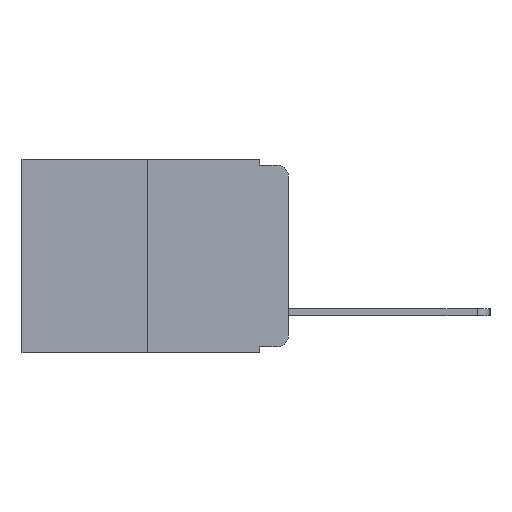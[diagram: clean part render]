
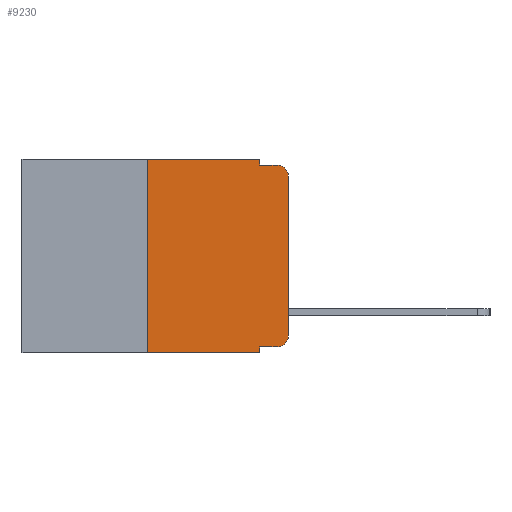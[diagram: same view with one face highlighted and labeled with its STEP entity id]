
A CAD part, left-side view. The second image highlights one B-rep face of the part: STEP entity #9230.
In plain terms, the highlighted planar face has unit normal (-1, 0, 0).
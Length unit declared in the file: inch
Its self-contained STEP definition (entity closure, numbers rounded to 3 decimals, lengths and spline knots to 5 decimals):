
#603 = VECTOR ( 'NONE', #9681, 39.37008 ) ;
#700 = AXIS2_PLACEMENT_3D ( 'NONE', #1759, #1698, #7909 ) ;
#852 = EDGE_CURVE ( 'NONE', #17246, #5633, #21928, .T. ) ;
#853 = CARTESIAN_POINT ( 'NONE',  ( 0., 0.051, -0.333 ) ) ;
#1263 = LINE ( 'NONE', #16762, #5682 ) ;
#1351 = VERTEX_POINT ( 'NONE', #10596 ) ;
#1698 = DIRECTION ( 'NONE',  ( -1., 0., 0. ) ) ;
#1759 = CARTESIAN_POINT ( 'NONE',  ( 0., 0.02, -0.313 ) ) ;
#2240 = EDGE_CURVE ( 'NONE', #18007, #17246, #8905, .T. ) ;
#2505 = LINE ( 'NONE', #14826, #11472 ) ;
#2826 = VERTEX_POINT ( 'NONE', #3504 ) ;
#2918 = LINE ( 'NONE', #5590, #16963 ) ;
#3504 = CARTESIAN_POINT ( 'NONE',  ( 0., 0.051, -0.343 ) ) ;
#3516 = EDGE_CURVE ( 'NONE', #18007, #2826, #2918, .T. ) ;
#4063 = ORIENTED_EDGE ( 'NONE', *, *, #4723, .F. ) ;
#4288 = DIRECTION ( 'NONE',  ( 0., -1., 0. ) ) ;
#4389 = CARTESIAN_POINT ( 'NONE',  ( 0., 0.25, -0.343 ) ) ;
#4510 = DIRECTION ( 'NONE',  ( 0., 0., 1. ) ) ;
#4723 = EDGE_CURVE ( 'NONE', #5943, #1351, #1263, .T. ) ;
#4977 = VERTEX_POINT ( 'NONE', #5205 ) ;
#5091 = ORIENTED_EDGE ( 'NONE', *, *, #3516, .F. ) ;
#5205 = CARTESIAN_POINT ( 'NONE',  ( 0., 0.051, -0.01 ) ) ;
#5473 = VERTEX_POINT ( 'NONE', #18615 ) ;
#5590 = CARTESIAN_POINT ( 'NONE',  ( 0., 0.051, 0. ) ) ;
#5633 = VERTEX_POINT ( 'NONE', #17326 ) ;
#5682 = VECTOR ( 'NONE', #4510, 39.37008 ) ;
#5930 = EDGE_CURVE ( 'NONE', #6834, #4977, #14478, .T. ) ;
#5943 = VERTEX_POINT ( 'NONE', #4389 ) ;
#6155 = CARTESIAN_POINT ( 'NONE',  ( 0., 0.473, 0. ) ) ;
#6527 = EDGE_CURVE ( 'NONE', #1351, #6834, #2505, .T. ) ;
#6761 = CARTESIAN_POINT ( 'NONE',  ( 0., 0.051, 0. ) ) ;
#6834 = VERTEX_POINT ( 'NONE', #6761 ) ;
#7132 = EDGE_CURVE ( 'NONE', #4977, #5473, #13359, .T. ) ;
#7755 = LINE ( 'NONE', #14783, #11308 ) ;
#7909 = DIRECTION ( 'NONE',  ( 0., 0., -1. ) ) ;
#7927 = CARTESIAN_POINT ( 'NONE',  ( 0., 0.051, 0. ) ) ;
#8905 = LINE ( 'NONE', #10770, #22115 ) ;
#9230 = ADVANCED_FACE ( 'NONE', ( #16764 ), #9718, .F. ) ;
#9500 = EDGE_CURVE ( 'NONE', #19135, #5473, #15961, .T. ) ;
#9546 = ORIENTED_EDGE ( 'NONE', *, *, #10684, .T. ) ;
#9681 = DIRECTION ( 'NONE',  ( 0., 0., -1. ) ) ;
#9716 = AXIS2_PLACEMENT_3D ( 'NONE', #6155, #16610, #13245 ) ;
#9718 = PLANE ( 'NONE',  #9716 ) ;
#10596 = CARTESIAN_POINT ( 'NONE',  ( 0., 0.25, 0. ) ) ;
#10634 = CARTESIAN_POINT ( 'NONE',  ( 0., 0.02, -0.03 ) ) ;
#10684 = EDGE_CURVE ( 'NONE', #5633, #19135, #7755, .T. ) ;
#10770 = CARTESIAN_POINT ( 'NONE',  ( 0., 0.051, -0.333 ) ) ;
#11092 = ORIENTED_EDGE ( 'NONE', *, *, #6527, .F. ) ;
#11097 = CARTESIAN_POINT ( 'NONE',  ( 0., 0.051, -0.01 ) ) ;
#11308 = VECTOR ( 'NONE', #19980, 39.37008 ) ;
#11472 = VECTOR ( 'NONE', #4288, 39.37008 ) ;
#11956 = AXIS2_PLACEMENT_3D ( 'NONE', #10634, #22652, #12406 ) ;
#12045 = CARTESIAN_POINT ( 'NONE',  ( 0., 0., -0.03 ) ) ;
#12286 = ORIENTED_EDGE ( 'NONE', *, *, #7132, .F. ) ;
#12404 = ORIENTED_EDGE ( 'NONE', *, *, #20670, .T. ) ;
#12406 = DIRECTION ( 'NONE',  ( 0., 0., -1. ) ) ;
#12463 = DIRECTION ( 'NONE',  ( 0., -1., 0. ) ) ;
#13245 = DIRECTION ( 'NONE',  ( 0., 0., -1. ) ) ;
#13359 = LINE ( 'NONE', #11097, #17365 ) ;
#14478 = LINE ( 'NONE', #7927, #603 ) ;
#14783 = CARTESIAN_POINT ( 'NONE',  ( 0., 0., 0. ) ) ;
#14826 = CARTESIAN_POINT ( 'NONE',  ( 0., 0.473, 0. ) ) ;
#15715 = ORIENTED_EDGE ( 'NONE', *, *, #2240, .T. ) ;
#15961 = CIRCLE ( 'NONE', #11956, 0.02 ) ;
#16610 = DIRECTION ( 'NONE',  ( 1., 0., 0. ) ) ;
#16762 = CARTESIAN_POINT ( 'NONE',  ( 0., 0.25, 0. ) ) ;
#16764 = FACE_OUTER_BOUND ( 'NONE', #21266, .T. ) ;
#16963 = VECTOR ( 'NONE', #17800, 39.37008 ) ;
#17246 = VERTEX_POINT ( 'NONE', #20098 ) ;
#17326 = CARTESIAN_POINT ( 'NONE',  ( 0., 0., -0.313 ) ) ;
#17365 = VECTOR ( 'NONE', #19773, 39.37008 ) ;
#17800 = DIRECTION ( 'NONE',  ( 0., 0., -1. ) ) ;
#18007 = VERTEX_POINT ( 'NONE', #853 ) ;
#18615 = CARTESIAN_POINT ( 'NONE',  ( 0., 0.02, -0.01 ) ) ;
#18846 = ORIENTED_EDGE ( 'NONE', *, *, #9500, .T. ) ;
#19135 = VERTEX_POINT ( 'NONE', #12045 ) ;
#19692 = ORIENTED_EDGE ( 'NONE', *, *, #5930, .F. ) ;
#19773 = DIRECTION ( 'NONE',  ( 0., -1., 0. ) ) ;
#19829 = CARTESIAN_POINT ( 'NONE',  ( 0., 0.473, -0.343 ) ) ;
#19980 = DIRECTION ( 'NONE',  ( 0., 0., 1. ) ) ;
#20098 = CARTESIAN_POINT ( 'NONE',  ( 0., 0.02, -0.333 ) ) ;
#20665 = VECTOR ( 'NONE', #21541, 39.37008 ) ;
#20670 = EDGE_CURVE ( 'NONE', #5943, #2826, #21203, .T. ) ;
#21203 = LINE ( 'NONE', #19829, #20665 ) ;
#21266 = EDGE_LOOP ( 'NONE', ( #9546, #18846, #12286, #19692, #11092, #4063, #12404, #5091, #15715, #22680 ) ) ;
#21541 = DIRECTION ( 'NONE',  ( 0., -1., 0. ) ) ;
#21928 = CIRCLE ( 'NONE', #700, 0.02 ) ;
#22115 = VECTOR ( 'NONE', #12463, 39.37008 ) ;
#22652 = DIRECTION ( 'NONE',  ( -1., 0., 0. ) ) ;
#22680 = ORIENTED_EDGE ( 'NONE', *, *, #852, .T. ) ;
